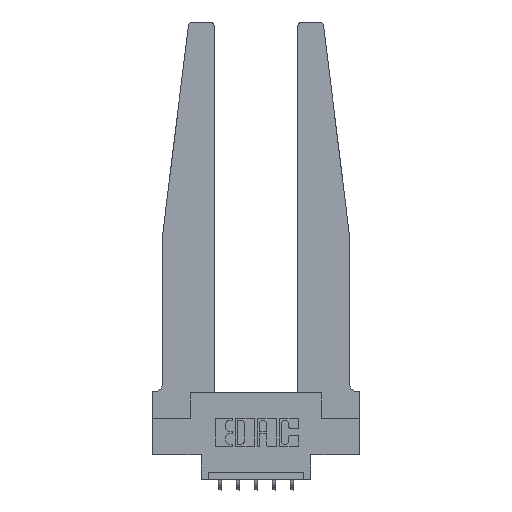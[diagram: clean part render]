
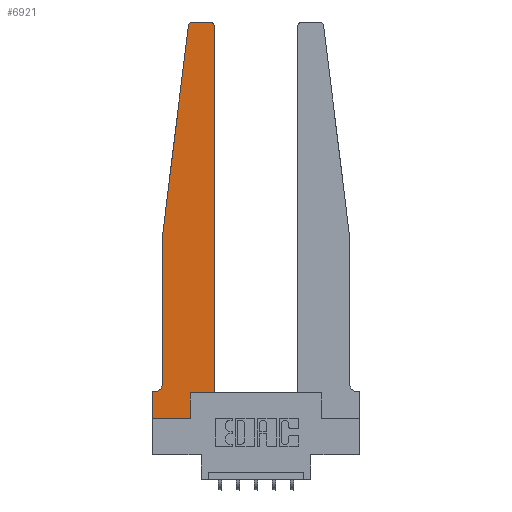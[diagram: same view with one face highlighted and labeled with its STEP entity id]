
A CAD part, top view. The second image highlights one B-rep face of the part: STEP entity #6921.
In plain terms, the highlighted planar face has unit normal (0, 0, 1).
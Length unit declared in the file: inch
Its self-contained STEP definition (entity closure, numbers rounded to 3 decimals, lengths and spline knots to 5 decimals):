
#27 = CARTESIAN_POINT ( 'NONE',  ( 0.27653, 2.75, 0.37 ) ) ;
#156 = VERTEX_POINT ( 'NONE', #747 ) ;
#231 = VECTOR ( 'NONE', #1201, 39.37008 ) ;
#375 = LINE ( 'NONE', #2344, #4808 ) ;
#511 = EDGE_CURVE ( 'NONE', #2948, #6632, #375, .T. ) ;
#608 = DIRECTION ( 'NONE',  ( 0., 0., -1. ) ) ;
#747 = CARTESIAN_POINT ( 'NONE',  ( 0.2605, 0.18, 0.37 ) ) ;
#785 = DIRECTION ( 'NONE',  ( 1., 0., 0. ) ) ;
#797 = DIRECTION ( 'NONE',  ( -1., 0., 0. ) ) ;
#829 = VECTOR ( 'NONE', #11198, 39.37008 ) ;
#892 = PLANE ( 'NONE',  #4932 ) ;
#1013 = CARTESIAN_POINT ( 'NONE',  ( 0., 0., 0.37 ) ) ;
#1201 = DIRECTION ( 'NONE',  ( 1., 0., 0. ) ) ;
#1283 = VERTEX_POINT ( 'NONE', #6602 ) ;
#1346 = CARTESIAN_POINT ( 'NONE',  ( 0.065, 0.1875, 0.37 ) ) ;
#1354 = EDGE_CURVE ( 'NONE', #11662, #10730, #11587, .T. ) ;
#1445 = AXIS2_PLACEMENT_3D ( 'NONE', #3580, #4737, #12042 ) ;
#1459 = DIRECTION ( 'NONE',  ( -0.122, -0.992, 0. ) ) ;
#1493 = CIRCLE ( 'NONE', #11513, 0.03 ) ;
#1671 = CARTESIAN_POINT ( 'NONE',  ( 0.395, 2.72, 0.37 ) ) ;
#1713 = CARTESIAN_POINT ( 'NONE',  ( 0.065, 1.25, 0.37 ) ) ;
#1796 = CARTESIAN_POINT ( 'NONE',  ( 0., 0.1875, 0.37 ) ) ;
#1801 = DIRECTION ( 'NONE',  ( 0., 0., 1. ) ) ;
#2329 = EDGE_CURVE ( 'NONE', #156, #2948, #4500, .T. ) ;
#2344 = CARTESIAN_POINT ( 'NONE',  ( 0.425, 0.18, 0.37 ) ) ;
#2477 = CARTESIAN_POINT ( 'NONE',  ( 0.065, 1.25, 0.37 ) ) ;
#2948 = VERTEX_POINT ( 'NONE', #7338 ) ;
#3021 = CARTESIAN_POINT ( 'NONE',  ( 0.25, 2.75, 0.37 ) ) ;
#3128 = EDGE_CURVE ( 'NONE', #6632, #7304, #1493, .T. ) ;
#3169 = LINE ( 'NONE', #5358, #231 ) ;
#3496 = DIRECTION ( 'NONE',  ( 0., 1., 0. ) ) ;
#3580 = CARTESIAN_POINT ( 'NONE',  ( 0.27653, 2.72, 0.37 ) ) ;
#3655 = VECTOR ( 'NONE', #10499, 39.37008 ) ;
#3946 = LINE ( 'NONE', #11326, #12871 ) ;
#4303 = ORIENTED_EDGE ( 'NONE', *, *, #9420, .T. ) ;
#4386 = CARTESIAN_POINT ( 'NONE',  ( 0.425, 2.72, 0.37 ) ) ;
#4429 = CARTESIAN_POINT ( 'NONE',  ( 0.015, 0.2375, 0.37 ) ) ;
#4433 = CARTESIAN_POINT ( 'NONE',  ( 0.425, 0.18, 0.37 ) ) ;
#4500 = LINE ( 'NONE', #4433, #5709 ) ;
#4737 = DIRECTION ( 'NONE',  ( 0., 0., 1. ) ) ;
#4808 = VECTOR ( 'NONE', #5486, 39.37008 ) ;
#4932 = AXIS2_PLACEMENT_3D ( 'NONE', #12354, #8111, #5045 ) ;
#4953 = VERTEX_POINT ( 'NONE', #27 ) ;
#5045 = DIRECTION ( 'NONE',  ( 1., 0., 0. ) ) ;
#5267 = EDGE_CURVE ( 'NONE', #5967, #9852, #3946, .T. ) ;
#5358 = CARTESIAN_POINT ( 'NONE',  ( 0., 0., 0.37 ) ) ;
#5486 = DIRECTION ( 'NONE',  ( 0., 1., 0. ) ) ;
#5709 = VECTOR ( 'NONE', #11806, 39.37008 ) ;
#5710 = EDGE_CURVE ( 'NONE', #9852, #1283, #3169, .T. ) ;
#5967 = VERTEX_POINT ( 'NONE', #1796 ) ;
#6602 = CARTESIAN_POINT ( 'NONE',  ( 0.2605, 0., 0.37 ) ) ;
#6632 = VERTEX_POINT ( 'NONE', #4386 ) ;
#6695 = EDGE_CURVE ( 'NONE', #1283, #156, #9506, .T. ) ;
#6921 = ADVANCED_FACE ( 'NONE', ( #9151 ), #892, .T. ) ;
#7128 = CARTESIAN_POINT ( 'NONE',  ( 0.065, 0.2375, 0.37 ) ) ;
#7178 = DIRECTION ( 'NONE',  ( -1., 0., 0. ) ) ;
#7304 = VERTEX_POINT ( 'NONE', #12266 ) ;
#7338 = CARTESIAN_POINT ( 'NONE',  ( 0.425, 0.18, 0.37 ) ) ;
#7483 = EDGE_CURVE ( 'NONE', #10730, #5967, #9466, .T. ) ;
#7683 = ORIENTED_EDGE ( 'NONE', *, *, #13498, .T. ) ;
#7995 = CARTESIAN_POINT ( 'NONE',  ( 0.015, 0.1875, 0.37 ) ) ;
#8032 = EDGE_CURVE ( 'NONE', #11146, #11662, #10106, .T. ) ;
#8111 = DIRECTION ( 'NONE',  ( 0., 0., 1. ) ) ;
#8191 = ORIENTED_EDGE ( 'NONE', *, *, #7483, .T. ) ;
#8321 = ORIENTED_EDGE ( 'NONE', *, *, #5267, .T. ) ;
#8369 = ORIENTED_EDGE ( 'NONE', *, *, #2329, .T. ) ;
#8765 = ORIENTED_EDGE ( 'NONE', *, *, #5710, .T. ) ;
#9016 = ORIENTED_EDGE ( 'NONE', *, *, #3128, .T. ) ;
#9124 = VECTOR ( 'NONE', #3496, 39.37008 ) ;
#9136 = DIRECTION ( 'NONE',  ( 0., -1., 0. ) ) ;
#9151 = FACE_OUTER_BOUND ( 'NONE', #9963, .T. ) ;
#9360 = ORIENTED_EDGE ( 'NONE', *, *, #8032, .T. ) ;
#9420 = EDGE_CURVE ( 'NONE', #4953, #10758, #12344, .T. ) ;
#9466 = LINE ( 'NONE', #1346, #3655 ) ;
#9506 = LINE ( 'NONE', #9705, #9124 ) ;
#9536 = ORIENTED_EDGE ( 'NONE', *, *, #511, .T. ) ;
#9705 = CARTESIAN_POINT ( 'NONE',  ( 0.2605, 0.18, 0.37 ) ) ;
#9852 = VERTEX_POINT ( 'NONE', #1013 ) ;
#9963 = EDGE_LOOP ( 'NONE', ( #11716, #4303, #7683, #9360, #9982, #8191, #8321, #8765, #11102, #8369, #9536, #9016 ) ) ;
#9982 = ORIENTED_EDGE ( 'NONE', *, *, #1354, .T. ) ;
#10045 = CARTESIAN_POINT ( 'NONE',  ( 0.065, 1.25, 0.37 ) ) ;
#10059 = CARTESIAN_POINT ( 'NONE',  ( 0.24675, 2.72367, 0.37 ) ) ;
#10106 = LINE ( 'NONE', #1713, #829 ) ;
#10372 = VECTOR ( 'NONE', #1459, 39.37008 ) ;
#10499 = DIRECTION ( 'NONE',  ( -1., 0., 0. ) ) ;
#10730 = VERTEX_POINT ( 'NONE', #7995 ) ;
#10758 = VERTEX_POINT ( 'NONE', #10059 ) ;
#10964 = EDGE_CURVE ( 'NONE', #7304, #4953, #12372, .T. ) ;
#11102 = ORIENTED_EDGE ( 'NONE', *, *, #6695, .T. ) ;
#11146 = VERTEX_POINT ( 'NONE', #10045 ) ;
#11198 = DIRECTION ( 'NONE',  ( 0., -1., 0. ) ) ;
#11326 = CARTESIAN_POINT ( 'NONE',  ( 0., 0., 0.37 ) ) ;
#11513 = AXIS2_PLACEMENT_3D ( 'NONE', #1671, #1801, #785 ) ;
#11587 = CIRCLE ( 'NONE', #13329, 0.05 ) ;
#11662 = VERTEX_POINT ( 'NONE', #7128 ) ;
#11716 = ORIENTED_EDGE ( 'NONE', *, *, #10964, .T. ) ;
#11806 = DIRECTION ( 'NONE',  ( 1., 0., 0. ) ) ;
#12042 = DIRECTION ( 'NONE',  ( 1., 0., 0. ) ) ;
#12266 = CARTESIAN_POINT ( 'NONE',  ( 0.395, 2.75, 0.37 ) ) ;
#12344 = CIRCLE ( 'NONE', #1445, 0.03 ) ;
#12354 = CARTESIAN_POINT ( 'NONE',  ( 0., 0.1875, 0.37 ) ) ;
#12372 = LINE ( 'NONE', #3021, #13181 ) ;
#12869 = LINE ( 'NONE', #2477, #10372 ) ;
#12871 = VECTOR ( 'NONE', #9136, 39.37008 ) ;
#13181 = VECTOR ( 'NONE', #7178, 39.37008 ) ;
#13329 = AXIS2_PLACEMENT_3D ( 'NONE', #4429, #608, #797 ) ;
#13498 = EDGE_CURVE ( 'NONE', #10758, #11146, #12869, .T. ) ;
